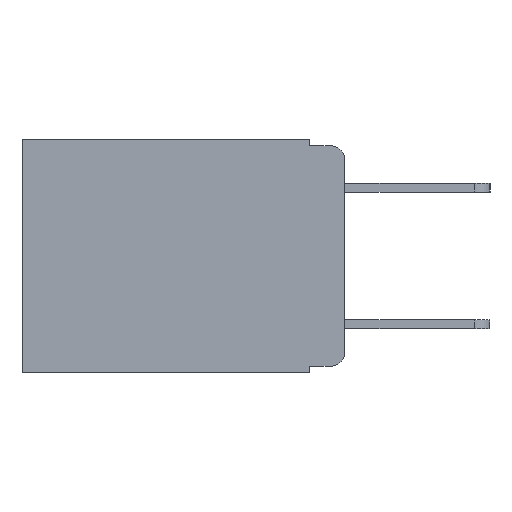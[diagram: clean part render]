
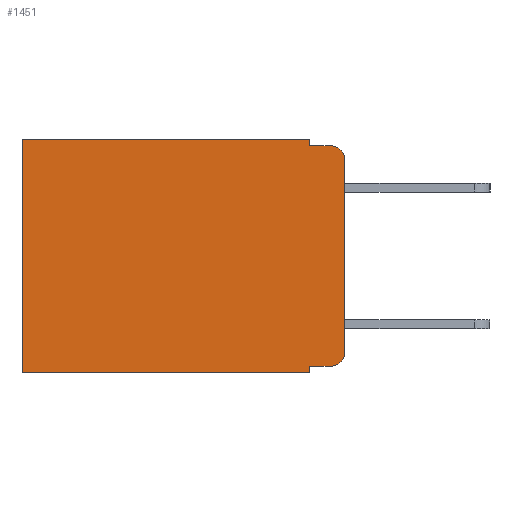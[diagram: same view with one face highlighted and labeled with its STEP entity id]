
A CAD part, left-side view. The second image highlights one B-rep face of the part: STEP entity #1451.
In plain terms, the highlighted planar face has unit normal (-1, 0, 0).
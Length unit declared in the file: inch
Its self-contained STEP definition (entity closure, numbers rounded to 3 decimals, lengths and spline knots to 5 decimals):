
#293 = AXIS2_PLACEMENT_3D ( 'NONE', #9618, #2056, #10705 ) ;
#352 = DIRECTION ( 'NONE',  ( 0., 0., -1. ) ) ;
#415 = DIRECTION ( 'NONE',  ( 0., 0., -1. ) ) ;
#442 = ORIENTED_EDGE ( 'NONE', *, *, #11354, .F. ) ;
#1191 = EDGE_CURVE ( 'NONE', #4763, #6974, #14534, .T. ) ;
#1451 = ADVANCED_FACE ( 'NONE', ( #1476 ), #6490, .F. ) ;
#1476 = FACE_OUTER_BOUND ( 'NONE', #7473, .T. ) ;
#2056 = DIRECTION ( 'NONE',  ( -1., 0., 0. ) ) ;
#2173 = VERTEX_POINT ( 'NONE', #14250 ) ;
#2694 = ORIENTED_EDGE ( 'NONE', *, *, #12174, .T. ) ;
#2705 = VERTEX_POINT ( 'NONE', #10500 ) ;
#2762 = CARTESIAN_POINT ( 'NONE',  ( 0.298, 0.051, -0.343 ) ) ;
#2808 = CARTESIAN_POINT ( 'NONE',  ( 0.298, 0.473, 0. ) ) ;
#3515 = CARTESIAN_POINT ( 'NONE',  ( 0.298, 0., 0. ) ) ;
#3634 = VERTEX_POINT ( 'NONE', #6039 ) ;
#3907 = CIRCLE ( 'NONE', #11515, 0.02 ) ;
#4347 = LINE ( 'NONE', #12514, #12819 ) ;
#4442 = CARTESIAN_POINT ( 'NONE',  ( 0.298, 0.051, -0.01 ) ) ;
#4763 = VERTEX_POINT ( 'NONE', #5608 ) ;
#4873 = VERTEX_POINT ( 'NONE', #13546 ) ;
#4890 = CARTESIAN_POINT ( 'NONE',  ( 0.298, 0.051, -0.01 ) ) ;
#5084 = DIRECTION ( 'NONE',  ( 0., 1., 0. ) ) ;
#5439 = ORIENTED_EDGE ( 'NONE', *, *, #12076, .T. ) ;
#5520 = CARTESIAN_POINT ( 'NONE',  ( 0.298, 0., 0. ) ) ;
#5608 = CARTESIAN_POINT ( 'NONE',  ( 0.298, 0.051, 0. ) ) ;
#5865 = VECTOR ( 'NONE', #12679, 39.37008 ) ;
#6001 = CARTESIAN_POINT ( 'NONE',  ( 0.298, 0.051, -0.333 ) ) ;
#6039 = CARTESIAN_POINT ( 'NONE',  ( 0.298, 0.02, -0.01 ) ) ;
#6252 = VERTEX_POINT ( 'NONE', #4890 ) ;
#6256 = LINE ( 'NONE', #8356, #9077 ) ;
#6382 = DIRECTION ( 'NONE',  ( 0., 0., -1. ) ) ;
#6490 = PLANE ( 'NONE',  #10155 ) ;
#6829 = ORIENTED_EDGE ( 'NONE', *, *, #11977, .F. ) ;
#6974 = VERTEX_POINT ( 'NONE', #2808 ) ;
#6977 = VERTEX_POINT ( 'NONE', #2762 ) ;
#7060 = DIRECTION ( 'NONE',  ( 0., 0., -1. ) ) ;
#7199 = DIRECTION ( 'NONE',  ( 0., 0., -1. ) ) ;
#7473 = EDGE_LOOP ( 'NONE', ( #14586, #14867, #6829, #12650, #15156, #12930, #442, #7924, #5439, #2694 ) ) ;
#7924 = ORIENTED_EDGE ( 'NONE', *, *, #12030, .F. ) ;
#8289 = DIRECTION ( 'NONE',  ( -1., 0., 0. ) ) ;
#8356 = CARTESIAN_POINT ( 'NONE',  ( 0.298, 0.051, 0. ) ) ;
#8446 = VECTOR ( 'NONE', #14167, 39.37008 ) ;
#8791 = CARTESIAN_POINT ( 'NONE',  ( 0.298, 0., -0.343 ) ) ;
#9077 = VECTOR ( 'NONE', #14551, 39.37008 ) ;
#9095 = VECTOR ( 'NONE', #5084, 39.37008 ) ;
#9394 = DIRECTION ( 'NONE',  ( 0., -1., 0. ) ) ;
#9412 = VECTOR ( 'NONE', #415, 39.37008 ) ;
#9618 = CARTESIAN_POINT ( 'NONE',  ( 0.298, 0.02, -0.313 ) ) ;
#9728 = VECTOR ( 'NONE', #9394, 39.37008 ) ;
#9842 = VERTEX_POINT ( 'NONE', #11905 ) ;
#9858 = DIRECTION ( 'NONE',  ( 1., 0., 0. ) ) ;
#10155 = AXIS2_PLACEMENT_3D ( 'NONE', #5520, #9858, #6382 ) ;
#10402 = LINE ( 'NONE', #4442, #9728 ) ;
#10500 = CARTESIAN_POINT ( 'NONE',  ( 0.298, 0.02, -0.333 ) ) ;
#10705 = DIRECTION ( 'NONE',  ( 0., 0., -1. ) ) ;
#11354 = EDGE_CURVE ( 'NONE', #6977, #4873, #11916, .T. ) ;
#11515 = AXIS2_PLACEMENT_3D ( 'NONE', #14467, #8289, #352 ) ;
#11592 = LINE ( 'NONE', #6001, #5865 ) ;
#11905 = CARTESIAN_POINT ( 'NONE',  ( 0.298, 0., -0.313 ) ) ;
#11916 = LINE ( 'NONE', #8791, #9095 ) ;
#11938 = EDGE_CURVE ( 'NONE', #12107, #9842, #4347, .T. ) ;
#11976 = EDGE_CURVE ( 'NONE', #12107, #3634, #3907, .T. ) ;
#11977 = EDGE_CURVE ( 'NONE', #6252, #3634, #10402, .T. ) ;
#11995 = EDGE_CURVE ( 'NONE', #4763, #6252, #14756, .T. ) ;
#12011 = EDGE_CURVE ( 'NONE', #6974, #4873, #14458, .T. ) ;
#12030 = EDGE_CURVE ( 'NONE', #2173, #6977, #6256, .T. ) ;
#12076 = EDGE_CURVE ( 'NONE', #2173, #2705, #11592, .T. ) ;
#12107 = VERTEX_POINT ( 'NONE', #14594 ) ;
#12174 = EDGE_CURVE ( 'NONE', #2705, #9842, #13881, .T. ) ;
#12232 = VECTOR ( 'NONE', #7199, 39.37008 ) ;
#12514 = CARTESIAN_POINT ( 'NONE',  ( 0.298, 0., 0. ) ) ;
#12650 = ORIENTED_EDGE ( 'NONE', *, *, #11995, .F. ) ;
#12679 = DIRECTION ( 'NONE',  ( 0., -1., 0. ) ) ;
#12819 = VECTOR ( 'NONE', #7060, 39.37008 ) ;
#12930 = ORIENTED_EDGE ( 'NONE', *, *, #12011, .T. ) ;
#13546 = CARTESIAN_POINT ( 'NONE',  ( 0.298, 0.473, -0.343 ) ) ;
#13599 = CARTESIAN_POINT ( 'NONE',  ( 0.298, 0.473, 0. ) ) ;
#13881 = CIRCLE ( 'NONE', #293, 0.02 ) ;
#14167 = DIRECTION ( 'NONE',  ( 0., 1., 0. ) ) ;
#14250 = CARTESIAN_POINT ( 'NONE',  ( 0.298, 0.051, -0.333 ) ) ;
#14458 = LINE ( 'NONE', #13599, #12232 ) ;
#14467 = CARTESIAN_POINT ( 'NONE',  ( 0.298, 0.02, -0.03 ) ) ;
#14506 = CARTESIAN_POINT ( 'NONE',  ( 0.298, 0.051, 0. ) ) ;
#14534 = LINE ( 'NONE', #3515, #8446 ) ;
#14551 = DIRECTION ( 'NONE',  ( 0., 0., -1. ) ) ;
#14586 = ORIENTED_EDGE ( 'NONE', *, *, #11938, .F. ) ;
#14594 = CARTESIAN_POINT ( 'NONE',  ( 0.298, 0., -0.03 ) ) ;
#14756 = LINE ( 'NONE', #14506, #9412 ) ;
#14867 = ORIENTED_EDGE ( 'NONE', *, *, #11976, .T. ) ;
#15156 = ORIENTED_EDGE ( 'NONE', *, *, #1191, .T. ) ;
